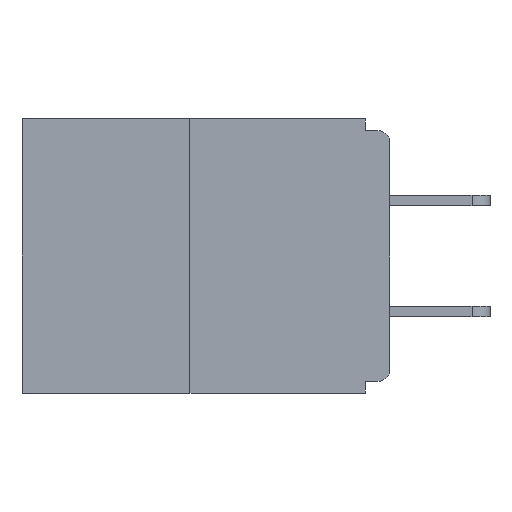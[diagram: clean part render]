
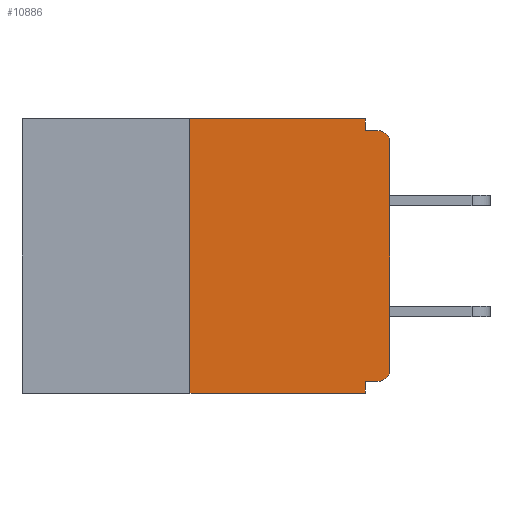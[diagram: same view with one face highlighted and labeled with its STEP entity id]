
A CAD part, left-side view. The second image highlights one B-rep face of the part: STEP entity #10886.
In plain terms, the highlighted planar face has unit normal (-1, 0, 0).
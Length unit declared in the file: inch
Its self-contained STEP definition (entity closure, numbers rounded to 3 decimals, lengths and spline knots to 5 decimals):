
#244 = CARTESIAN_POINT ( 'NONE',  ( 0., 0.031, -0.015 ) ) ;
#385 = CARTESIAN_POINT ( 'NONE',  ( 0., 0.46, -0.343 ) ) ;
#400 = VERTEX_POINT ( 'NONE', #11709 ) ;
#468 = CARTESIAN_POINT ( 'NONE',  ( 0., 0.25, 0. ) ) ;
#828 = EDGE_CURVE ( 'NONE', #8102, #4558, #2398, .T. ) ;
#1221 = CARTESIAN_POINT ( 'NONE',  ( 0., 0.015, -0.03 ) ) ;
#1258 = FACE_OUTER_BOUND ( 'NONE', #9379, .T. ) ;
#1345 = DIRECTION ( 'NONE',  ( 0., 0., -1. ) ) ;
#1486 = VERTEX_POINT ( 'NONE', #4586 ) ;
#1523 = LINE ( 'NONE', #468, #2469 ) ;
#1610 = CARTESIAN_POINT ( 'NONE',  ( 0., 0.031, 0. ) ) ;
#1819 = DIRECTION ( 'NONE',  ( 0., 0., -1. ) ) ;
#1882 = DIRECTION ( 'NONE',  ( 0., 1., 0. ) ) ;
#2398 = LINE ( 'NONE', #12537, #2686 ) ;
#2469 = VECTOR ( 'NONE', #11182, 39.37008 ) ;
#2686 = VECTOR ( 'NONE', #1882, 39.37008 ) ;
#2724 = CARTESIAN_POINT ( 'NONE',  ( 0., 0.031, -0.343 ) ) ;
#3135 = DIRECTION ( 'NONE',  ( -1., 0., 0. ) ) ;
#3448 = LINE ( 'NONE', #12565, #4665 ) ;
#3453 = AXIS2_PLACEMENT_3D ( 'NONE', #4967, #4885, #11637 ) ;
#3518 = ORIENTED_EDGE ( 'NONE', *, *, #8291, .F. ) ;
#3650 = LINE ( 'NONE', #6958, #12333 ) ;
#4065 = CARTESIAN_POINT ( 'NONE',  ( 0., 0., -0.313 ) ) ;
#4072 = VECTOR ( 'NONE', #8419, 39.37008 ) ;
#4194 = DIRECTION ( 'NONE',  ( -1., 0., 0. ) ) ;
#4236 = CARTESIAN_POINT ( 'NONE',  ( 0., 0.015, -0.313 ) ) ;
#4413 = CIRCLE ( 'NONE', #11344, 0.015 ) ;
#4558 = VERTEX_POINT ( 'NONE', #6057 ) ;
#4586 = CARTESIAN_POINT ( 'NONE',  ( 0., 0.25, -0.343 ) ) ;
#4665 = VECTOR ( 'NONE', #1819, 39.37008 ) ;
#4869 = ORIENTED_EDGE ( 'NONE', *, *, #9790, .F. ) ;
#4871 = EDGE_CURVE ( 'NONE', #10194, #9389, #3448, .T. ) ;
#4885 = DIRECTION ( 'NONE',  ( 1., 0., 0. ) ) ;
#4967 = CARTESIAN_POINT ( 'NONE',  ( 0., 0.46, 0. ) ) ;
#5015 = EDGE_CURVE ( 'NONE', #8102, #9277, #6000, .T. ) ;
#5428 = CARTESIAN_POINT ( 'NONE',  ( 0., 0.015, -0.328 ) ) ;
#5739 = VECTOR ( 'NONE', #11009, 39.37008 ) ;
#5792 = CARTESIAN_POINT ( 'NONE',  ( 0., 0.031, -0.343 ) ) ;
#5887 = CARTESIAN_POINT ( 'NONE',  ( 0., 0.25, 0. ) ) ;
#5892 = LINE ( 'NONE', #9962, #5739 ) ;
#6000 = CIRCLE ( 'NONE', #9199, 0.015 ) ;
#6057 = CARTESIAN_POINT ( 'NONE',  ( 0., 0.031, -0.328 ) ) ;
#6327 = EDGE_CURVE ( 'NONE', #9277, #400, #9951, .T. ) ;
#6487 = DIRECTION ( 'NONE',  ( 0., 0., 1. ) ) ;
#6693 = LINE ( 'NONE', #2724, #9611 ) ;
#6819 = VERTEX_POINT ( 'NONE', #5887 ) ;
#6958 = CARTESIAN_POINT ( 'NONE',  ( 0., 0.46, 0. ) ) ;
#7954 = ORIENTED_EDGE ( 'NONE', *, *, #5015, .T. ) ;
#8054 = EDGE_CURVE ( 'NONE', #1486, #6819, #1523, .T. ) ;
#8102 = VERTEX_POINT ( 'NONE', #5428 ) ;
#8291 = EDGE_CURVE ( 'NONE', #4558, #10875, #6693, .T. ) ;
#8419 = DIRECTION ( 'NONE',  ( 0., -1., 0. ) ) ;
#8517 = VERTEX_POINT ( 'NONE', #10935 ) ;
#8693 = EDGE_CURVE ( 'NONE', #6819, #10194, #3650, .T. ) ;
#8770 = ORIENTED_EDGE ( 'NONE', *, *, #4871, .F. ) ;
#8885 = VECTOR ( 'NONE', #6487, 39.37008 ) ;
#9193 = ORIENTED_EDGE ( 'NONE', *, *, #8054, .F. ) ;
#9199 = AXIS2_PLACEMENT_3D ( 'NONE', #4236, #4194, #1345 ) ;
#9277 = VERTEX_POINT ( 'NONE', #4065 ) ;
#9379 = EDGE_LOOP ( 'NONE', ( #11424, #9193, #11871, #3518, #12303, #7954, #9737, #11220, #4869, #8770 ) ) ;
#9389 = VERTEX_POINT ( 'NONE', #244 ) ;
#9611 = VECTOR ( 'NONE', #10394, 39.37008 ) ;
#9737 = ORIENTED_EDGE ( 'NONE', *, *, #6327, .T. ) ;
#9751 = EDGE_CURVE ( 'NONE', #400, #8517, #4413, .T. ) ;
#9790 = EDGE_CURVE ( 'NONE', #9389, #8517, #5892, .T. ) ;
#9951 = LINE ( 'NONE', #12326, #8885 ) ;
#9962 = CARTESIAN_POINT ( 'NONE',  ( 0., 0., -0.015 ) ) ;
#10181 = EDGE_CURVE ( 'NONE', #1486, #10875, #11838, .T. ) ;
#10194 = VERTEX_POINT ( 'NONE', #1610 ) ;
#10394 = DIRECTION ( 'NONE',  ( 0., 0., -1. ) ) ;
#10617 = PLANE ( 'NONE',  #3453 ) ;
#10875 = VERTEX_POINT ( 'NONE', #5792 ) ;
#10877 = DIRECTION ( 'NONE',  ( 0., -1., 0. ) ) ;
#10886 = ADVANCED_FACE ( 'NONE', ( #1258 ), #10617, .F. ) ;
#10935 = CARTESIAN_POINT ( 'NONE',  ( 0., 0.015, -0.015 ) ) ;
#11009 = DIRECTION ( 'NONE',  ( 0., -1., 0. ) ) ;
#11109 = DIRECTION ( 'NONE',  ( 0., 0., -1. ) ) ;
#11182 = DIRECTION ( 'NONE',  ( 0., 0., 1. ) ) ;
#11220 = ORIENTED_EDGE ( 'NONE', *, *, #9751, .T. ) ;
#11344 = AXIS2_PLACEMENT_3D ( 'NONE', #1221, #3135, #11109 ) ;
#11424 = ORIENTED_EDGE ( 'NONE', *, *, #8693, .F. ) ;
#11637 = DIRECTION ( 'NONE',  ( 0., 0., -1. ) ) ;
#11709 = CARTESIAN_POINT ( 'NONE',  ( 0., 0., -0.03 ) ) ;
#11838 = LINE ( 'NONE', #385, #4072 ) ;
#11871 = ORIENTED_EDGE ( 'NONE', *, *, #10181, .T. ) ;
#12303 = ORIENTED_EDGE ( 'NONE', *, *, #828, .F. ) ;
#12326 = CARTESIAN_POINT ( 'NONE',  ( 0., 0., 0. ) ) ;
#12333 = VECTOR ( 'NONE', #10877, 39.37008 ) ;
#12537 = CARTESIAN_POINT ( 'NONE',  ( 0., 0., -0.328 ) ) ;
#12565 = CARTESIAN_POINT ( 'NONE',  ( 0., 0.031, 0. ) ) ;
